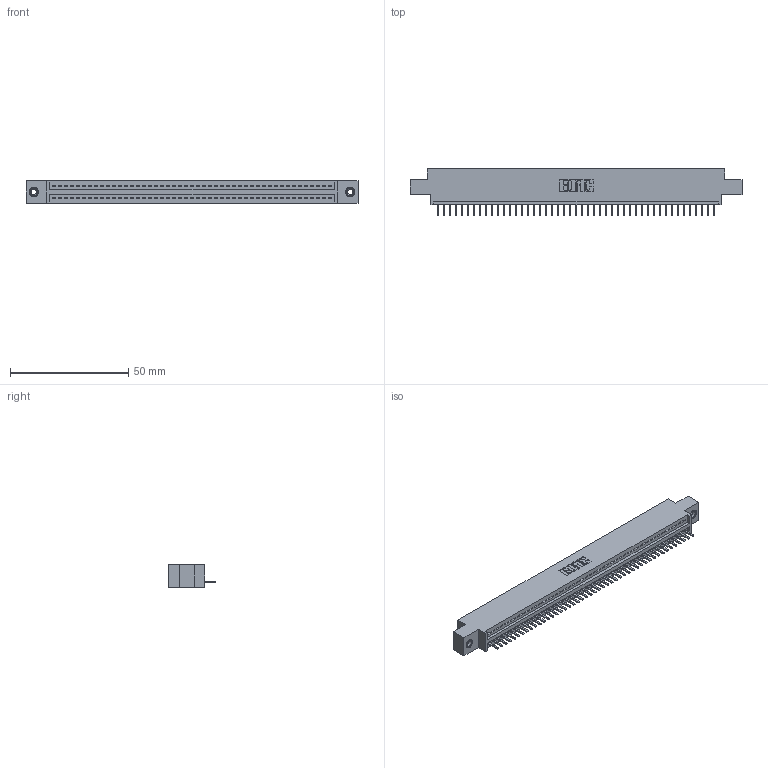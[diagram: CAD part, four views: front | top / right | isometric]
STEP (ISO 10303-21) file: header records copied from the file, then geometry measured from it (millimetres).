
FILE_DESCRIPTION (( 'STEP AP203' ), '1' );
FILE_NAME ('395-047-520-608.STEP', '2019-10-22T22:51:22', ( '' ), ( '' ), 'SwSTEP 2.0', 'SolidWorks 2016', '' );
FILE_SCHEMA (( 'CONFIG_CONTROL_DESIGN' ));
Length unit declared in the file: inch
Products named in the file (4): 345-250-001_345-250-003-102; 395-047-520-608; 345 Part_0.170 Offset - 0.156 Dia-TI; 345-292-001_345-293-120
Assembly tree (50 placements, depth 2):
  395-047-520-608
    345 Part_0.170 Offset - 0.156 Dia-TI
    345-292-001_345-293-120  x47
    345-250-001_345-250-003-102  x2
Bounding box: 140.59 x 19.68 x 9.4 mm (x, y, z)
Volume: 13139.1 mm3; surface area: 17232.1 mm2
Topology: 50 solids, 50 shells, 3104 faces, 9137 edges, 5958 vertices
Faces by surface type: plane 2090, cylinder 998, cone 12, torus 4
Entity records: 36132 total; most frequent: CARTESIAN_POINT 6252, ORIENTED_EDGE 6214, DIRECTION 5467, EDGE_CURVE 3107, VECTOR 2763, LINE 2763, VERTEX_POINT 2064, AXIS2_PLACEMENT_3D 1352
